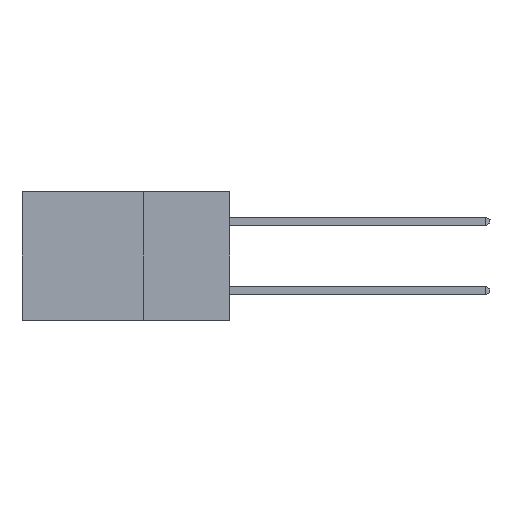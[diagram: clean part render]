
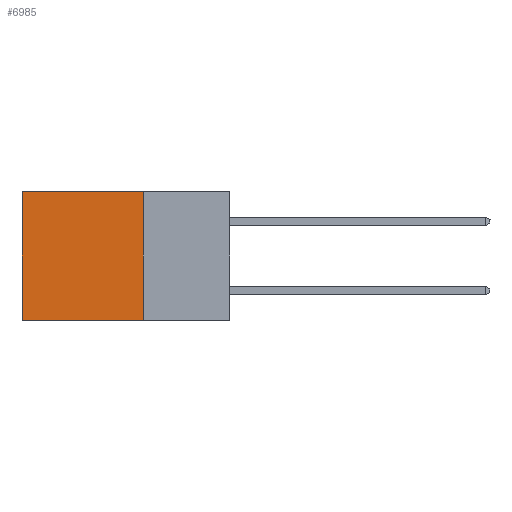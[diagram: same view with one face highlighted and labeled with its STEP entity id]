
A CAD part, left-side view. The second image highlights one B-rep face of the part: STEP entity #6985.
In plain terms, the highlighted planar face has unit normal (-1, 0, 0).
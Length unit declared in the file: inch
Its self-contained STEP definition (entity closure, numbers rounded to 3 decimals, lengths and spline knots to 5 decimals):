
#284 = VERTEX_POINT ( 'NONE', #10635 ) ;
#425 = EDGE_LOOP ( 'NONE', ( #2258, #9269, #5506, #2055 ) ) ;
#536 = CARTESIAN_POINT ( 'NONE',  ( 0.298, 0.25, 0. ) ) ;
#775 = AXIS2_PLACEMENT_3D ( 'NONE', #3111, #11294, #4145 ) ;
#1051 = VECTOR ( 'NONE', #1915, 39.37008 ) ;
#1134 = LINE ( 'NONE', #8640, #2424 ) ;
#1915 = DIRECTION ( 'NONE',  ( 0., 1., 0. ) ) ;
#2055 = ORIENTED_EDGE ( 'NONE', *, *, #8792, .T. ) ;
#2258 = ORIENTED_EDGE ( 'NONE', *, *, #6185, .T. ) ;
#2424 = VECTOR ( 'NONE', #9593, 39.37008 ) ;
#3003 = VECTOR ( 'NONE', #8122, 39.37008 ) ;
#3084 = CARTESIAN_POINT ( 'NONE',  ( 0.298, 0.6, 0. ) ) ;
#3111 = CARTESIAN_POINT ( 'NONE',  ( 0.298, 0.25, 0. ) ) ;
#4023 = VERTEX_POINT ( 'NONE', #536 ) ;
#4145 = DIRECTION ( 'NONE',  ( 0., 0., -1. ) ) ;
#4770 = EDGE_CURVE ( 'NONE', #4023, #9243, #1134, .T. ) ;
#5046 = CARTESIAN_POINT ( 'NONE',  ( 0.298, 0.25, -0.37 ) ) ;
#5506 = ORIENTED_EDGE ( 'NONE', *, *, #4770, .F. ) ;
#5821 = LINE ( 'NONE', #6971, #1051 ) ;
#6177 = DIRECTION ( 'NONE',  ( 0., 0., -1. ) ) ;
#6185 = EDGE_CURVE ( 'NONE', #284, #12564, #11994, .T. ) ;
#6971 = CARTESIAN_POINT ( 'NONE',  ( 0.298, 0.25, 0. ) ) ;
#6985 = ADVANCED_FACE ( 'NONE', ( #10051 ), #9197, .F. ) ;
#7745 = EDGE_CURVE ( 'NONE', #9243, #12564, #11796, .T. ) ;
#8122 = DIRECTION ( 'NONE',  ( 0., 1., 0. ) ) ;
#8640 = CARTESIAN_POINT ( 'NONE',  ( 0.298, 0.25, 0. ) ) ;
#8792 = EDGE_CURVE ( 'NONE', #4023, #284, #5821, .T. ) ;
#9197 = PLANE ( 'NONE',  #775 ) ;
#9243 = VERTEX_POINT ( 'NONE', #11825 ) ;
#9269 = ORIENTED_EDGE ( 'NONE', *, *, #7745, .F. ) ;
#9593 = DIRECTION ( 'NONE',  ( 0., 0., -1. ) ) ;
#10051 = FACE_OUTER_BOUND ( 'NONE', #425, .T. ) ;
#10587 = VECTOR ( 'NONE', #6177, 39.37008 ) ;
#10635 = CARTESIAN_POINT ( 'NONE',  ( 0.298, 0.6, 0. ) ) ;
#11294 = DIRECTION ( 'NONE',  ( 1., 0., 0. ) ) ;
#11796 = LINE ( 'NONE', #5046, #3003 ) ;
#11825 = CARTESIAN_POINT ( 'NONE',  ( 0.298, 0.25, -0.37 ) ) ;
#11994 = LINE ( 'NONE', #3084, #10587 ) ;
#12424 = CARTESIAN_POINT ( 'NONE',  ( 0.298, 0.6, -0.37 ) ) ;
#12564 = VERTEX_POINT ( 'NONE', #12424 ) ;
